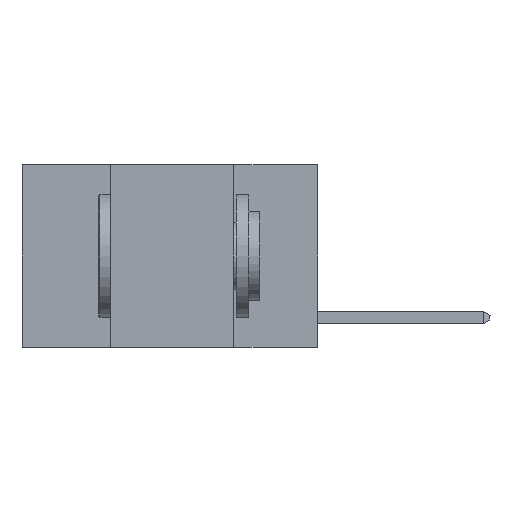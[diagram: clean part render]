
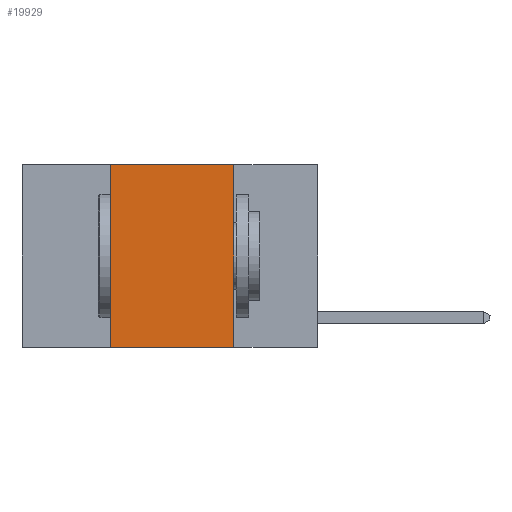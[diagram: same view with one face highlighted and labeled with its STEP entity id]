
A CAD part, left-side view. The second image highlights one B-rep face of the part: STEP entity #19929.
In plain terms, the highlighted planar face has unit normal (-1, 0, 0).
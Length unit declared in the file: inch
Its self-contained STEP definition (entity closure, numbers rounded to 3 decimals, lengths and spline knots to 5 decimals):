
#1176 = DIRECTION ( 'NONE',  ( 0., 0., 1. ) ) ;
#1254 = VERTEX_POINT ( 'NONE', #11358 ) ;
#2319 = EDGE_CURVE ( 'NONE', #27833, #1254, #26589, .T. ) ;
#3528 = CARTESIAN_POINT ( 'NONE',  ( 0., 0.6, 0. ) ) ;
#3995 = ORIENTED_EDGE ( 'NONE', *, *, #22872, .T. ) ;
#5893 = DIRECTION ( 'NONE',  ( 1., 0., 0. ) ) ;
#6145 = LINE ( 'NONE', #14281, #17899 ) ;
#6332 = DIRECTION ( 'NONE',  ( 0., -1., 0. ) ) ;
#7668 = DIRECTION ( 'NONE',  ( 0., -1., 0. ) ) ;
#9157 = EDGE_CURVE ( 'NONE', #18847, #27833, #24437, .T. ) ;
#9881 = VECTOR ( 'NONE', #1176, 39.37008 ) ;
#11358 = CARTESIAN_POINT ( 'NONE',  ( 0., 0.17, 0. ) ) ;
#13350 = CARTESIAN_POINT ( 'NONE',  ( 0., 0.6, 0. ) ) ;
#14211 = VECTOR ( 'NONE', #6332, 39.37008 ) ;
#14218 = VECTOR ( 'NONE', #7668, 39.37008 ) ;
#14281 = CARTESIAN_POINT ( 'NONE',  ( 0., 0.17, 0. ) ) ;
#16232 = CARTESIAN_POINT ( 'NONE',  ( 0., 0.42, -0.37 ) ) ;
#17249 = ORIENTED_EDGE ( 'NONE', *, *, #21619, .F. ) ;
#17604 = PLANE ( 'NONE',  #20421 ) ;
#17899 = VECTOR ( 'NONE', #28209, 39.37008 ) ;
#18847 = VERTEX_POINT ( 'NONE', #16232 ) ;
#19310 = CARTESIAN_POINT ( 'NONE',  ( 0., 0.6, -0.37 ) ) ;
#19929 = ADVANCED_FACE ( 'NONE', ( #23757 ), #17604, .F. ) ;
#20421 = AXIS2_PLACEMENT_3D ( 'NONE', #3528, #5893, #22254 ) ;
#20671 = EDGE_LOOP ( 'NONE', ( #17249, #23139, #26057, #3995 ) ) ;
#21619 = EDGE_CURVE ( 'NONE', #1254, #25855, #6145, .T. ) ;
#22254 = DIRECTION ( 'NONE',  ( 0., 0., -1. ) ) ;
#22872 = EDGE_CURVE ( 'NONE', #18847, #25855, #25848, .T. ) ;
#23139 = ORIENTED_EDGE ( 'NONE', *, *, #2319, .F. ) ;
#23757 = FACE_OUTER_BOUND ( 'NONE', #20671, .T. ) ;
#24437 = LINE ( 'NONE', #26945, #9881 ) ;
#25848 = LINE ( 'NONE', #19310, #14218 ) ;
#25855 = VERTEX_POINT ( 'NONE', #28610 ) ;
#26057 = ORIENTED_EDGE ( 'NONE', *, *, #9157, .F. ) ;
#26589 = LINE ( 'NONE', #13350, #14211 ) ;
#26945 = CARTESIAN_POINT ( 'NONE',  ( 0., 0.42, 0. ) ) ;
#27399 = CARTESIAN_POINT ( 'NONE',  ( 0., 0.42, 0. ) ) ;
#27833 = VERTEX_POINT ( 'NONE', #27399 ) ;
#28209 = DIRECTION ( 'NONE',  ( 0., 0., -1. ) ) ;
#28610 = CARTESIAN_POINT ( 'NONE',  ( 0., 0.17, -0.37 ) ) ;
